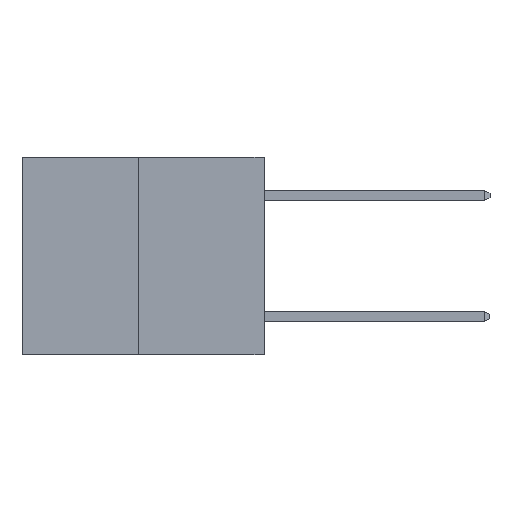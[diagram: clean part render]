
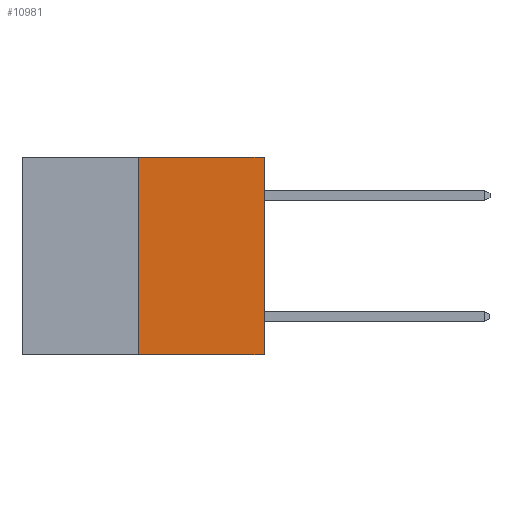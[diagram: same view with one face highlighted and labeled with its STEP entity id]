
A CAD part, left-side view. The second image highlights one B-rep face of the part: STEP entity #10981.
In plain terms, the highlighted planar face has unit normal (-1, 0, 0).
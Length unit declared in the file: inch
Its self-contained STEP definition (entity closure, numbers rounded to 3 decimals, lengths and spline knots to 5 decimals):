
#534 = CARTESIAN_POINT ( 'NONE',  ( 0., 0., -0.49 ) ) ;
#803 = VECTOR ( 'NONE', #7692, 39.37008 ) ;
#983 = VECTOR ( 'NONE', #1886, 39.37008 ) ;
#997 = DIRECTION ( 'NONE',  ( 1., 0., 0. ) ) ;
#1886 = DIRECTION ( 'NONE',  ( 0., 0., 1. ) ) ;
#2837 = VERTEX_POINT ( 'NONE', #8012 ) ;
#3127 = VERTEX_POINT ( 'NONE', #4560 ) ;
#3271 = CARTESIAN_POINT ( 'NONE',  ( 0., 0.6, 0. ) ) ;
#3314 = ORIENTED_EDGE ( 'NONE', *, *, #17342, .F. ) ;
#3991 = EDGE_CURVE ( 'NONE', #13987, #11787, #12370, .T. ) ;
#4560 = CARTESIAN_POINT ( 'NONE',  ( 0., 0.312, -0.49 ) ) ;
#6202 = DIRECTION ( 'NONE',  ( 0., 0., 1. ) ) ;
#7668 = CARTESIAN_POINT ( 'NONE',  ( 0., 0., 0. ) ) ;
#7692 = DIRECTION ( 'NONE',  ( 0., -1., 0. ) ) ;
#7817 = VECTOR ( 'NONE', #11546, 39.37008 ) ;
#7936 = VECTOR ( 'NONE', #6202, 39.37008 ) ;
#8012 = CARTESIAN_POINT ( 'NONE',  ( 0., 0.312, 0. ) ) ;
#8265 = ORIENTED_EDGE ( 'NONE', *, *, #3991, .T. ) ;
#8881 = FACE_OUTER_BOUND ( 'NONE', #15588, .T. ) ;
#9766 = PLANE ( 'NONE',  #16279 ) ;
#10836 = LINE ( 'NONE', #3271, #803 ) ;
#10981 = ADVANCED_FACE ( 'NONE', ( #8881 ), #9766, .F. ) ;
#11546 = DIRECTION ( 'NONE',  ( 0., -1., 0. ) ) ;
#11787 = VERTEX_POINT ( 'NONE', #12930 ) ;
#12370 = LINE ( 'NONE', #7668, #983 ) ;
#12671 = ORIENTED_EDGE ( 'NONE', *, *, #14283, .T. ) ;
#12930 = CARTESIAN_POINT ( 'NONE',  ( 0., 0., 0. ) ) ;
#12971 = LINE ( 'NONE', #17200, #7817 ) ;
#13956 = DIRECTION ( 'NONE',  ( 0., 0., -1. ) ) ;
#13987 = VERTEX_POINT ( 'NONE', #534 ) ;
#14283 = EDGE_CURVE ( 'NONE', #3127, #13987, #12971, .T. ) ;
#14342 = ORIENTED_EDGE ( 'NONE', *, *, #17319, .F. ) ;
#14628 = LINE ( 'NONE', #14694, #7936 ) ;
#14694 = CARTESIAN_POINT ( 'NONE',  ( 0., 0.312, -0.49 ) ) ;
#15588 = EDGE_LOOP ( 'NONE', ( #3314, #12671, #8265, #14342 ) ) ;
#16279 = AXIS2_PLACEMENT_3D ( 'NONE', #18106, #997, #13956 ) ;
#17200 = CARTESIAN_POINT ( 'NONE',  ( 0., 0.6, -0.49 ) ) ;
#17319 = EDGE_CURVE ( 'NONE', #2837, #11787, #10836, .T. ) ;
#17342 = EDGE_CURVE ( 'NONE', #3127, #2837, #14628, .T. ) ;
#18106 = CARTESIAN_POINT ( 'NONE',  ( 0., 0.6, 0. ) ) ;
